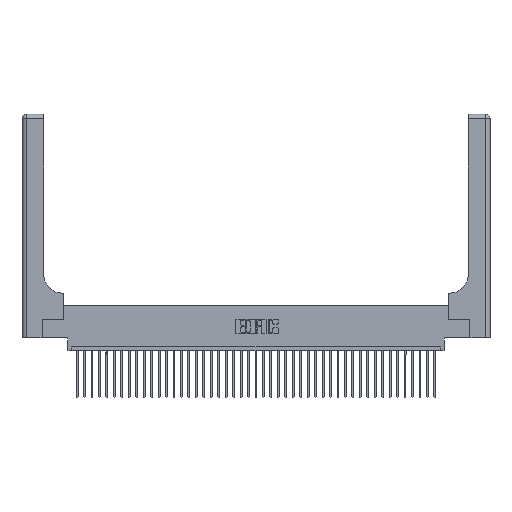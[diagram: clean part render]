
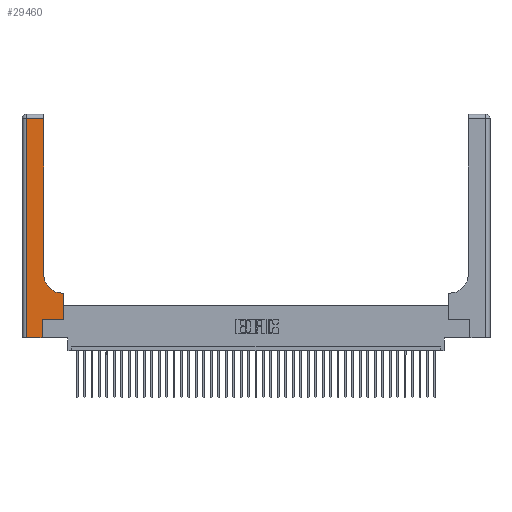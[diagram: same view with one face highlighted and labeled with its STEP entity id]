
A CAD part, top view. The second image highlights one B-rep face of the part: STEP entity #29460.
In plain terms, the highlighted planar face has unit normal (0, 0, 1).
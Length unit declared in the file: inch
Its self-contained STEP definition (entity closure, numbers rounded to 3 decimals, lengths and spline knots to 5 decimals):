
#202 = CARTESIAN_POINT ( 'NONE',  ( 0.5585, 0.25, 0.37 ) ) ;
#1190 = LINE ( 'NONE', #26588, #34097 ) ;
#1210 = CARTESIAN_POINT ( 'NONE',  ( 0.2915, 0.85, 0.37 ) ) ;
#1431 = VERTEX_POINT ( 'NONE', #16270 ) ;
#1533 = DIRECTION ( 'NONE',  ( 0., -1., 0. ) ) ;
#1594 = DIRECTION ( 'NONE',  ( 0., 1., 0. ) ) ;
#1885 = LINE ( 'NONE', #38019, #34750 ) ;
#2200 = LINE ( 'NONE', #17437, #17078 ) ;
#2324 = CIRCLE ( 'NONE', #26085, 0.25 ) ;
#2690 = DIRECTION ( 'NONE',  ( 1., 0., 0. ) ) ;
#2812 = CARTESIAN_POINT ( 'NONE',  ( 0., 0., 0.37 ) ) ;
#3195 = ORIENTED_EDGE ( 'NONE', *, *, #5068, .T. ) ;
#3244 = VECTOR ( 'NONE', #3388, 39.37008 ) ;
#3388 = DIRECTION ( 'NONE',  ( 0., 1., 0. ) ) ;
#3549 = CARTESIAN_POINT ( 'NONE',  ( 0., 3., 0.37 ) ) ;
#4559 = VECTOR ( 'NONE', #7438, 39.37008 ) ;
#5068 = EDGE_CURVE ( 'NONE', #21446, #35993, #1885, .T. ) ;
#5170 = VERTEX_POINT ( 'NONE', #29732 ) ;
#5273 = CARTESIAN_POINT ( 'NONE',  ( 0.5415, 0.6, 0.37 ) ) ;
#6478 = EDGE_CURVE ( 'NONE', #13443, #37467, #25157, .T. ) ;
#6677 = CARTESIAN_POINT ( 'NONE',  ( 0.5585, 0.6, 0.37 ) ) ;
#7438 = DIRECTION ( 'NONE',  ( -1., 0., 0. ) ) ;
#7825 = VERTEX_POINT ( 'NONE', #28988 ) ;
#8461 = LINE ( 'NONE', #14231, #36281 ) ;
#10110 = DIRECTION ( 'NONE',  ( -1., 0., 0. ) ) ;
#11512 = ORIENTED_EDGE ( 'NONE', *, *, #6478, .T. ) ;
#13443 = VERTEX_POINT ( 'NONE', #14035 ) ;
#13502 = CARTESIAN_POINT ( 'NONE',  ( 0.06, 2.94, 0.37 ) ) ;
#14035 = CARTESIAN_POINT ( 'NONE',  ( 0.06, 0., 0.37 ) ) ;
#14231 = CARTESIAN_POINT ( 'NONE',  ( 0.269, 0., 0.37 ) ) ;
#16270 = CARTESIAN_POINT ( 'NONE',  ( 0.2915, 2.94, 0.37 ) ) ;
#17078 = VECTOR ( 'NONE', #1594, 39.37008 ) ;
#17437 = CARTESIAN_POINT ( 'NONE',  ( 0.2915, 3., 0.37 ) ) ;
#17825 = DIRECTION ( 'NONE',  ( 0., 1., 0. ) ) ;
#18506 = VERTEX_POINT ( 'NONE', #1210 ) ;
#19570 = DIRECTION ( 'NONE',  ( 0., 0., -1. ) ) ;
#19706 = LINE ( 'NONE', #202, #3244 ) ;
#20110 = EDGE_LOOP ( 'NONE', ( #35742, #21201, #26978, #11512, #33052, #34551, #27979, #3195, #21542 ) ) ;
#20841 = DIRECTION ( 'NONE',  ( 1., 0., 0. ) ) ;
#21201 = ORIENTED_EDGE ( 'NONE', *, *, #24742, .T. ) ;
#21446 = VERTEX_POINT ( 'NONE', #6677 ) ;
#21542 = ORIENTED_EDGE ( 'NONE', *, *, #22443, .T. ) ;
#22364 = EDGE_CURVE ( 'NONE', #7825, #5170, #24729, .T. ) ;
#22443 = EDGE_CURVE ( 'NONE', #35993, #18506, #2324, .T. ) ;
#24729 = LINE ( 'NONE', #38027, #31194 ) ;
#24742 = EDGE_CURVE ( 'NONE', #1431, #34572, #34464, .T. ) ;
#25157 = LINE ( 'NONE', #2812, #39586 ) ;
#25971 = PLANE ( 'NONE',  #39979 ) ;
#26085 = AXIS2_PLACEMENT_3D ( 'NONE', #26404, #39227, #20841 ) ;
#26404 = CARTESIAN_POINT ( 'NONE',  ( 0.5415, 0.85, 0.37 ) ) ;
#26588 = CARTESIAN_POINT ( 'NONE',  ( 0.06, 3., 0.37 ) ) ;
#26978 = ORIENTED_EDGE ( 'NONE', *, *, #33045, .T. ) ;
#27979 = ORIENTED_EDGE ( 'NONE', *, *, #32233, .T. ) ;
#28988 = CARTESIAN_POINT ( 'NONE',  ( 0.269, 0.25, 0.37 ) ) ;
#29460 = ADVANCED_FACE ( 'NONE', ( #33928 ), #25971, .F. ) ;
#29732 = CARTESIAN_POINT ( 'NONE',  ( 0.5585, 0.25, 0.37 ) ) ;
#31188 = DIRECTION ( 'NONE',  ( -1., 0., 0. ) ) ;
#31194 = VECTOR ( 'NONE', #40713, 39.37008 ) ;
#32233 = EDGE_CURVE ( 'NONE', #5170, #21446, #19706, .T. ) ;
#32343 = CARTESIAN_POINT ( 'NONE',  ( 0., 2.94, 0.37 ) ) ;
#33045 = EDGE_CURVE ( 'NONE', #34572, #13443, #1190, .T. ) ;
#33052 = ORIENTED_EDGE ( 'NONE', *, *, #40318, .T. ) ;
#33928 = FACE_OUTER_BOUND ( 'NONE', #20110, .T. ) ;
#34097 = VECTOR ( 'NONE', #1533, 39.37008 ) ;
#34181 = EDGE_CURVE ( 'NONE', #18506, #1431, #2200, .T. ) ;
#34245 = CARTESIAN_POINT ( 'NONE',  ( 0.269, 0., 0.37 ) ) ;
#34464 = LINE ( 'NONE', #32343, #4559 ) ;
#34551 = ORIENTED_EDGE ( 'NONE', *, *, #22364, .T. ) ;
#34572 = VERTEX_POINT ( 'NONE', #13502 ) ;
#34750 = VECTOR ( 'NONE', #31188, 39.37008 ) ;
#35742 = ORIENTED_EDGE ( 'NONE', *, *, #34181, .T. ) ;
#35993 = VERTEX_POINT ( 'NONE', #5273 ) ;
#36281 = VECTOR ( 'NONE', #17825, 39.37008 ) ;
#37467 = VERTEX_POINT ( 'NONE', #34245 ) ;
#38019 = CARTESIAN_POINT ( 'NONE',  ( 0.2915, 0.6, 0.37 ) ) ;
#38027 = CARTESIAN_POINT ( 'NONE',  ( 0.269, 0.25, 0.37 ) ) ;
#39227 = DIRECTION ( 'NONE',  ( 0., 0., -1. ) ) ;
#39586 = VECTOR ( 'NONE', #2690, 39.37008 ) ;
#39979 = AXIS2_PLACEMENT_3D ( 'NONE', #3549, #19570, #10110 ) ;
#40318 = EDGE_CURVE ( 'NONE', #37467, #7825, #8461, .T. ) ;
#40713 = DIRECTION ( 'NONE',  ( 1., 0., 0. ) ) ;
